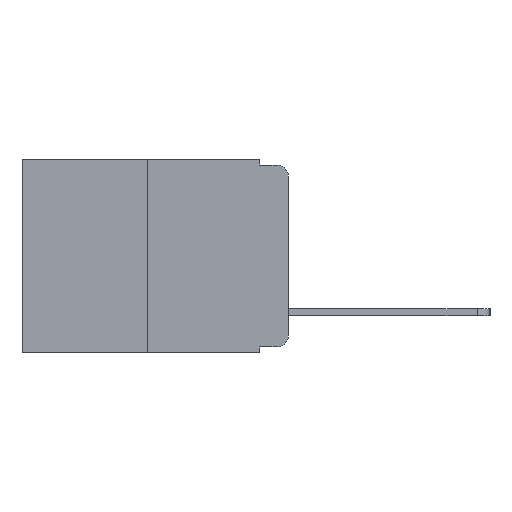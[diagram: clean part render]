
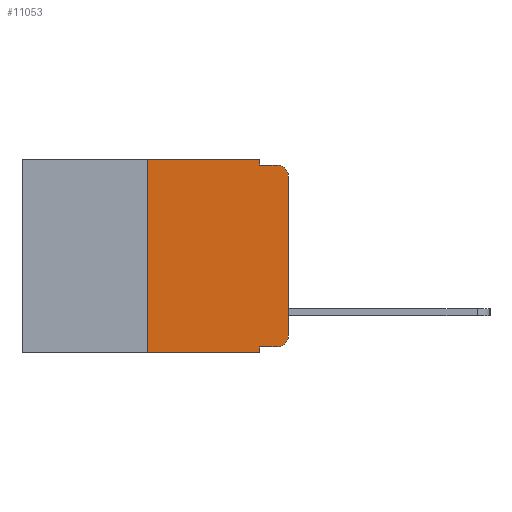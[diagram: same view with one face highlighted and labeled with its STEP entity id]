
A CAD part, left-side view. The second image highlights one B-rep face of the part: STEP entity #11053.
In plain terms, the highlighted planar face has unit normal (-1, 0, 0).
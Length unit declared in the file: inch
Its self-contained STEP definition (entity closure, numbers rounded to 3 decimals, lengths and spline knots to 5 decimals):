
#29 = EDGE_CURVE ( 'NONE', #4607, #8518, #3248, .T. ) ;
#294 = ORIENTED_EDGE ( 'NONE', *, *, #14707, .F. ) ;
#383 = CARTESIAN_POINT ( 'NONE',  ( 0., 0.25, 0. ) ) ;
#483 = CARTESIAN_POINT ( 'NONE',  ( 0., 0.473, 0. ) ) ;
#751 = CARTESIAN_POINT ( 'NONE',  ( 0., 0., -0.313 ) ) ;
#1091 = AXIS2_PLACEMENT_3D ( 'NONE', #2185, #13495, #3971 ) ;
#1135 = CARTESIAN_POINT ( 'NONE',  ( 0., 0., -0.03 ) ) ;
#1259 = EDGE_CURVE ( 'NONE', #7862, #5620, #17136, .T. ) ;
#1266 = LINE ( 'NONE', #16330, #5320 ) ;
#2185 = CARTESIAN_POINT ( 'NONE',  ( 0., 0.02, -0.313 ) ) ;
#2571 = ORIENTED_EDGE ( 'NONE', *, *, #13626, .F. ) ;
#2680 = VERTEX_POINT ( 'NONE', #11404 ) ;
#3104 = VECTOR ( 'NONE', #14812, 39.37008 ) ;
#3151 = ORIENTED_EDGE ( 'NONE', *, *, #8312, .T. ) ;
#3248 = CIRCLE ( 'NONE', #6499, 0.02 ) ;
#3281 = LINE ( 'NONE', #17656, #19627 ) ;
#3436 = LINE ( 'NONE', #10096, #7746 ) ;
#3813 = VECTOR ( 'NONE', #14482, 39.37008 ) ;
#3904 = ORIENTED_EDGE ( 'NONE', *, *, #15783, .F. ) ;
#3971 = DIRECTION ( 'NONE',  ( 0., 0., -1. ) ) ;
#4281 = CARTESIAN_POINT ( 'NONE',  ( 0., 0.473, -0.343 ) ) ;
#4607 = VERTEX_POINT ( 'NONE', #1135 ) ;
#4763 = EDGE_CURVE ( 'NONE', #6628, #4607, #3281, .T. ) ;
#4978 = CARTESIAN_POINT ( 'NONE',  ( 0., 0.051, 0. ) ) ;
#5227 = PLANE ( 'NONE',  #14891 ) ;
#5303 = VERTEX_POINT ( 'NONE', #12549 ) ;
#5320 = VECTOR ( 'NONE', #11644, 39.37008 ) ;
#5620 = VERTEX_POINT ( 'NONE', #14764 ) ;
#6442 = LINE ( 'NONE', #4281, #14383 ) ;
#6499 = AXIS2_PLACEMENT_3D ( 'NONE', #20833, #16624, #10723 ) ;
#6628 = VERTEX_POINT ( 'NONE', #751 ) ;
#6824 = DIRECTION ( 'NONE',  ( 0., 0., -1. ) ) ;
#7746 = VECTOR ( 'NONE', #19510, 39.37008 ) ;
#7862 = VERTEX_POINT ( 'NONE', #9195 ) ;
#7875 = VERTEX_POINT ( 'NONE', #17157 ) ;
#8181 = DIRECTION ( 'NONE',  ( 0., 0., 1. ) ) ;
#8203 = ORIENTED_EDGE ( 'NONE', *, *, #8461, .T. ) ;
#8312 = EDGE_CURVE ( 'NONE', #2680, #6628, #9378, .T. ) ;
#8461 = EDGE_CURVE ( 'NONE', #17948, #7875, #6442, .T. ) ;
#8518 = VERTEX_POINT ( 'NONE', #18492 ) ;
#9195 = CARTESIAN_POINT ( 'NONE',  ( 0., 0.25, 0. ) ) ;
#9342 = EDGE_CURVE ( 'NONE', #5303, #2680, #15892, .T. ) ;
#9378 = CIRCLE ( 'NONE', #1091, 0.02 ) ;
#10096 = CARTESIAN_POINT ( 'NONE',  ( 0., 0.051, -0.01 ) ) ;
#10723 = DIRECTION ( 'NONE',  ( 0., 0., -1. ) ) ;
#11053 = ADVANCED_FACE ( 'NONE', ( #11803 ), #5227, .F. ) ;
#11170 = ORIENTED_EDGE ( 'NONE', *, *, #1259, .F. ) ;
#11404 = CARTESIAN_POINT ( 'NONE',  ( 0., 0.02, -0.333 ) ) ;
#11452 = VERTEX_POINT ( 'NONE', #14152 ) ;
#11514 = EDGE_CURVE ( 'NONE', #5303, #7875, #16024, .T. ) ;
#11644 = DIRECTION ( 'NONE',  ( 0., 0., -1. ) ) ;
#11684 = VECTOR ( 'NONE', #18134, 39.37008 ) ;
#11803 = FACE_OUTER_BOUND ( 'NONE', #12739, .T. ) ;
#12549 = CARTESIAN_POINT ( 'NONE',  ( 0., 0.051, -0.333 ) ) ;
#12739 = EDGE_LOOP ( 'NONE', ( #20439, #18759, #3904, #294, #11170, #2571, #8203, #20725, #17608, #3151 ) ) ;
#13213 = CARTESIAN_POINT ( 'NONE',  ( 0., 0.051, -0.333 ) ) ;
#13495 = DIRECTION ( 'NONE',  ( -1., 0., 0. ) ) ;
#13626 = EDGE_CURVE ( 'NONE', #17948, #7862, #19508, .T. ) ;
#13649 = DIRECTION ( 'NONE',  ( 0., -1., 0. ) ) ;
#14152 = CARTESIAN_POINT ( 'NONE',  ( 0., 0.051, -0.01 ) ) ;
#14383 = VECTOR ( 'NONE', #16939, 39.37008 ) ;
#14482 = DIRECTION ( 'NONE',  ( 0., 0., -1. ) ) ;
#14640 = CARTESIAN_POINT ( 'NONE',  ( 0., 0.25, -0.343 ) ) ;
#14707 = EDGE_CURVE ( 'NONE', #5620, #11452, #1266, .T. ) ;
#14764 = CARTESIAN_POINT ( 'NONE',  ( 0., 0.051, 0. ) ) ;
#14812 = DIRECTION ( 'NONE',  ( 0., -1., 0. ) ) ;
#14891 = AXIS2_PLACEMENT_3D ( 'NONE', #20858, #16281, #6824 ) ;
#15783 = EDGE_CURVE ( 'NONE', #11452, #8518, #3436, .T. ) ;
#15892 = LINE ( 'NONE', #13213, #3104 ) ;
#16024 = LINE ( 'NONE', #4978, #3813 ) ;
#16281 = DIRECTION ( 'NONE',  ( 1., 0., 0. ) ) ;
#16330 = CARTESIAN_POINT ( 'NONE',  ( 0., 0.051, 0. ) ) ;
#16624 = DIRECTION ( 'NONE',  ( -1., 0., 0. ) ) ;
#16636 = VECTOR ( 'NONE', #13649, 39.37008 ) ;
#16939 = DIRECTION ( 'NONE',  ( 0., -1., 0. ) ) ;
#17136 = LINE ( 'NONE', #483, #16636 ) ;
#17157 = CARTESIAN_POINT ( 'NONE',  ( 0., 0.051, -0.343 ) ) ;
#17608 = ORIENTED_EDGE ( 'NONE', *, *, #9342, .T. ) ;
#17656 = CARTESIAN_POINT ( 'NONE',  ( 0., 0., 0. ) ) ;
#17948 = VERTEX_POINT ( 'NONE', #14640 ) ;
#18134 = DIRECTION ( 'NONE',  ( 0., 0., 1. ) ) ;
#18492 = CARTESIAN_POINT ( 'NONE',  ( 0., 0.02, -0.01 ) ) ;
#18759 = ORIENTED_EDGE ( 'NONE', *, *, #29, .T. ) ;
#19508 = LINE ( 'NONE', #383, #11684 ) ;
#19510 = DIRECTION ( 'NONE',  ( 0., -1., 0. ) ) ;
#19627 = VECTOR ( 'NONE', #8181, 39.37008 ) ;
#20439 = ORIENTED_EDGE ( 'NONE', *, *, #4763, .T. ) ;
#20725 = ORIENTED_EDGE ( 'NONE', *, *, #11514, .F. ) ;
#20833 = CARTESIAN_POINT ( 'NONE',  ( 0., 0.02, -0.03 ) ) ;
#20858 = CARTESIAN_POINT ( 'NONE',  ( 0., 0.473, 0. ) ) ;
